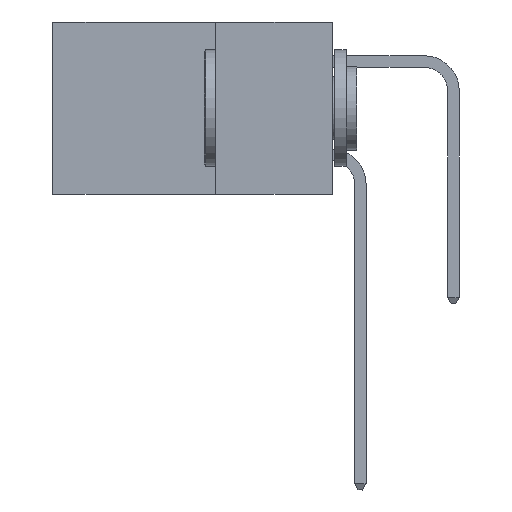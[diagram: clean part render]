
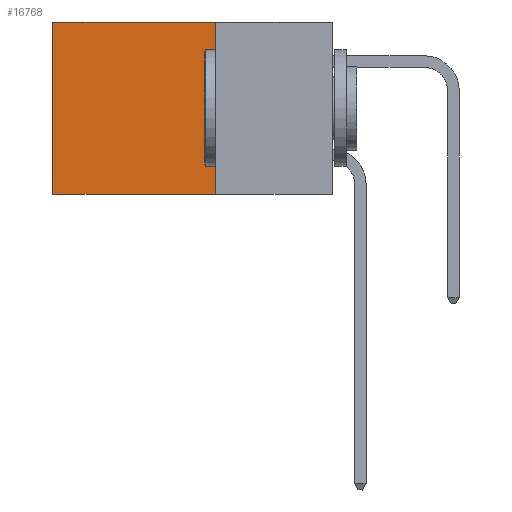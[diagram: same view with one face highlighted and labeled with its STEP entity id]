
A CAD part, left-side view. The second image highlights one B-rep face of the part: STEP entity #16768.
In plain terms, the highlighted planar face has unit normal (-1, 0, 0).
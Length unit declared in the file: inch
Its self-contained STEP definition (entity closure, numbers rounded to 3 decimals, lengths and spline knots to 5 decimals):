
#1021 = EDGE_CURVE ( 'NONE', #16182, #12039, #4359, .T. ) ;
#1763 = CARTESIAN_POINT ( 'NONE',  ( 0.298, 0.6, 0. ) ) ;
#1932 = CARTESIAN_POINT ( 'NONE',  ( 0.298, 0.25, -0.37 ) ) ;
#2394 = VECTOR ( 'NONE', #20326, 39.37008 ) ;
#3223 = VECTOR ( 'NONE', #12002, 39.37008 ) ;
#3951 = DIRECTION ( 'NONE',  ( 1., 0., 0. ) ) ;
#4359 = LINE ( 'NONE', #1932, #11633 ) ;
#7038 = CARTESIAN_POINT ( 'NONE',  ( 0.298, 0.25, 0. ) ) ;
#7371 = EDGE_CURVE ( 'NONE', #13732, #16182, #10690, .T. ) ;
#8145 = ORIENTED_EDGE ( 'NONE', *, *, #16673, .T. ) ;
#8950 = FACE_OUTER_BOUND ( 'NONE', #15450, .T. ) ;
#9255 = ORIENTED_EDGE ( 'NONE', *, *, #1021, .F. ) ;
#10145 = VECTOR ( 'NONE', #13364, 39.37008 ) ;
#10690 = LINE ( 'NONE', #20558, #2394 ) ;
#11633 = VECTOR ( 'NONE', #19520, 39.37008 ) ;
#12002 = DIRECTION ( 'NONE',  ( 0., 1., 0. ) ) ;
#12039 = VERTEX_POINT ( 'NONE', #21111 ) ;
#12065 = ORIENTED_EDGE ( 'NONE', *, *, #19216, .T. ) ;
#12389 = CARTESIAN_POINT ( 'NONE',  ( 0.298, 0.25, -0.37 ) ) ;
#13364 = DIRECTION ( 'NONE',  ( 0., 0., -1. ) ) ;
#13732 = VERTEX_POINT ( 'NONE', #20690 ) ;
#13922 = PLANE ( 'NONE',  #20792 ) ;
#14054 = LINE ( 'NONE', #1763, #10145 ) ;
#15450 = EDGE_LOOP ( 'NONE', ( #12065, #9255, #18718, #8145 ) ) ;
#15566 = CARTESIAN_POINT ( 'NONE',  ( 0.298, 0.25, 0. ) ) ;
#15633 = DIRECTION ( 'NONE',  ( 0., 0., -1. ) ) ;
#16182 = VERTEX_POINT ( 'NONE', #12389 ) ;
#16673 = EDGE_CURVE ( 'NONE', #13732, #18907, #19841, .T. ) ;
#16768 = ADVANCED_FACE ( 'NONE', ( #8950 ), #13922, .F. ) ;
#18718 = ORIENTED_EDGE ( 'NONE', *, *, #7371, .F. ) ;
#18907 = VERTEX_POINT ( 'NONE', #19193 ) ;
#19193 = CARTESIAN_POINT ( 'NONE',  ( 0.298, 0.6, 0. ) ) ;
#19216 = EDGE_CURVE ( 'NONE', #18907, #12039, #14054, .T. ) ;
#19520 = DIRECTION ( 'NONE',  ( 0., 1., 0. ) ) ;
#19841 = LINE ( 'NONE', #7038, #3223 ) ;
#20326 = DIRECTION ( 'NONE',  ( 0., 0., -1. ) ) ;
#20558 = CARTESIAN_POINT ( 'NONE',  ( 0.298, 0.25, 0. ) ) ;
#20690 = CARTESIAN_POINT ( 'NONE',  ( 0.298, 0.25, 0. ) ) ;
#20792 = AXIS2_PLACEMENT_3D ( 'NONE', #15566, #3951, #15633 ) ;
#21111 = CARTESIAN_POINT ( 'NONE',  ( 0.298, 0.6, -0.37 ) ) ;
